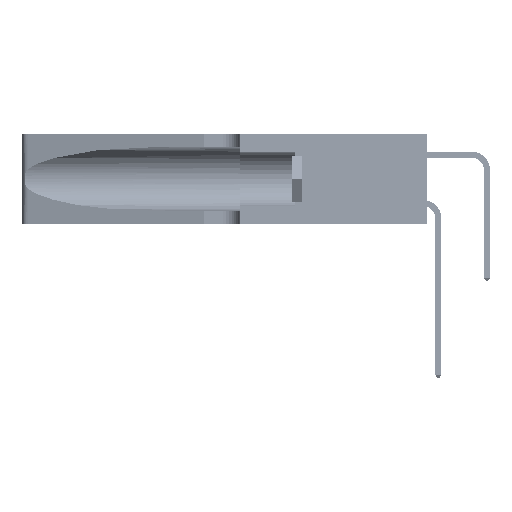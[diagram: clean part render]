
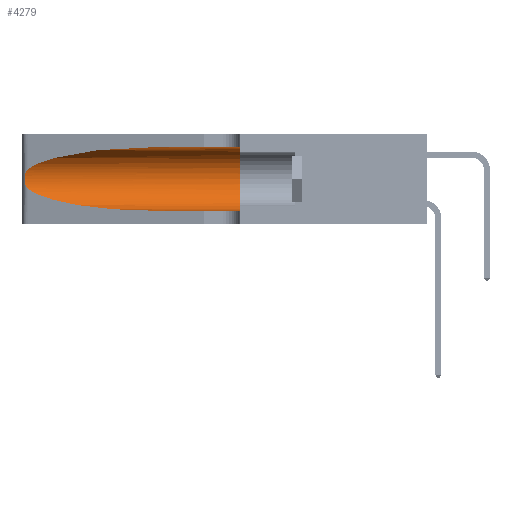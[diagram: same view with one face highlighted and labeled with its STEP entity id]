
A CAD part, left-side view. The second image highlights one B-rep face of the part: STEP entity #4279.
In plain terms, the highlighted cylindrical face has radius 3.308 mm (diameter 6.617 mm), a partial arc.
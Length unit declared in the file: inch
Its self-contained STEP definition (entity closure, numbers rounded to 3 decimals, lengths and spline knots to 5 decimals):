
#1733 = EDGE_CURVE ( 'NONE', #29096, #23608, #14990, .T. ) ;
#1966 = ORIENTED_EDGE ( 'NONE', *, *, #8866, .T. ) ;
#2706 = CARTESIAN_POINT ( 'NONE',  ( 0.25487, 1.22718, 0.22369 ) ) ;
#3504 = CARTESIAN_POINT ( 'NONE',  ( 0.25555, 1.22993, 0.14849 ) ) ;
#4279 = ADVANCED_FACE ( 'NONE', ( #16477 ), #40839, .F. ) ;
#5134 = CARTESIAN_POINT ( 'NONE',  ( 0.2373, 1.15595, 0.08982 ) ) ;
#5676 = CARTESIAN_POINT ( 'NONE',  ( 0.25487, 1.22718, 0.14631 ) ) ;
#7489 = CARTESIAN_POINT ( 'NONE',  ( 0.25487, 1.22718, 0.22369 ) ) ;
#8312 = CARTESIAN_POINT ( 'NONE',  ( 0.1305, 1.61858, 0.185 ) ) ;
#8866 = EDGE_CURVE ( 'NONE', #23500, #29096, #22328, .T. ) ;
#8928 = CARTESIAN_POINT ( 'NONE',  ( 0.1305, 0.72297, 0.05475 ) ) ;
#10269 = CARTESIAN_POINT ( 'NONE',  ( 0.25787, 1.23484, 0.2124 ) ) ;
#12177 = CARTESIAN_POINT ( 'NONE',  ( 0.1305, 0.35, 0.31525 ) ) ;
#12567 = CARTESIAN_POINT ( 'NONE',  ( 0.1305, 1.61858, 0.05475 ) ) ;
#12892 = VERTEX_POINT ( 'NONE', #12177 ) ;
#13508 = ORIENTED_EDGE ( 'NONE', *, *, #34425, .F. ) ;
#14007 = CARTESIAN_POINT ( 'NONE',  ( 0.1305, 1.61858, 0.31525 ) ) ;
#14303 = CARTESIAN_POINT ( 'NONE',  ( 0.1305, 0.35, 0.185 ) ) ;
#14594 = CARTESIAN_POINT ( 'NONE',  ( 0.26018, 1.23835, 0.19895 ) ) ;
#14990 = LINE ( 'NONE', #12567, #33189 ) ;
#16477 = FACE_OUTER_BOUND ( 'NONE', #47210, .T. ) ;
#16656 = VERTEX_POINT ( 'NONE', #23889 ) ;
#18002 = DIRECTION ( 'NONE',  ( 0., 0., 1. ) ) ;
#18304 = CARTESIAN_POINT ( 'NONE',  ( 0.26075, 1.23896, 0.178 ) ) ;
#19402 = DIRECTION ( 'NONE',  ( 0., 0., -1. ) ) ;
#21965 = CARTESIAN_POINT ( 'NONE',  ( 0.25856, 1.23593, 0.16098 ) ) ;
#22129 = CARTESIAN_POINT ( 'NONE',  ( 0.1305, 0.72297, 0.31525 ) ) ;
#22328 =( BOUNDED_CURVE ( )  B_SPLINE_CURVE ( 3, ( #30811, #5134, #23558, #8928 ),
 .UNSPECIFIED., .F., .T. ) 
 B_SPLINE_CURVE_WITH_KNOTS ( ( 4, 4 ),
 ( 3.44316, 4.71239 ),
 .UNSPECIFIED. ) 
 CURVE ( )  GEOMETRIC_REPRESENTATION_ITEM ( )  RATIONAL_B_SPLINE_CURVE ( ( 1., 0.87, 0.87, 1. ) ) 
 REPRESENTATION_ITEM ( '' )  );
#23151 = CARTESIAN_POINT ( 'NONE',  ( 0.25487, 1.22718, 0.22369 ) ) ;
#23500 = VERTEX_POINT ( 'NONE', #5676 ) ;
#23558 = CARTESIAN_POINT ( 'NONE',  ( 0.18966, 0.96281, 0.05475 ) ) ;
#23608 = VERTEX_POINT ( 'NONE', #28349 ) ;
#23634 = EDGE_CURVE ( 'NONE', #28376, #23500, #27299, .T. ) ;
#23889 = CARTESIAN_POINT ( 'NONE',  ( 0.1305, 0.72297, 0.31525 ) ) ;
#24861 = CARTESIAN_POINT ( 'NONE',  ( 0.25555, 1.22994, 0.2215 ) ) ;
#25637 = CARTESIAN_POINT ( 'NONE',  ( 0.25639, 1.23186, 0.15144 ) ) ;
#25801 = CARTESIAN_POINT ( 'NONE',  ( 0.18966, 0.96281, 0.31525 ) ) ;
#27299 = B_SPLINE_CURVE_WITH_KNOTS ( 'NONE', 3,
 ( #2706, #24861, #32103, #10269, #35726, #14594, #39980, #18304, #43600, #21965, #47193, #25637, #3504, #29287 ),
 .UNSPECIFIED., .F., .F.,
 ( 4, 2, 2, 2, 2, 2, 4 ),
 ( 0., 0.00027, 0.00053, 0.00107, 0.0016, 0.00187, 0.00214 ),
 .UNSPECIFIED. ) ;
#27392 = CARTESIAN_POINT ( 'NONE',  ( 0.1305, 0.72297, 0.05475 ) ) ;
#28349 = CARTESIAN_POINT ( 'NONE',  ( 0.1305, 0.35, 0.05475 ) ) ;
#28376 = VERTEX_POINT ( 'NONE', #23151 ) ;
#29096 = VERTEX_POINT ( 'NONE', #27392 ) ;
#29287 = CARTESIAN_POINT ( 'NONE',  ( 0.25487, 1.22718, 0.14631 ) ) ;
#29330 = VECTOR ( 'NONE', #39397, 39.37008 ) ;
#29403 = ORIENTED_EDGE ( 'NONE', *, *, #37634, .F. ) ;
#29426 = CARTESIAN_POINT ( 'NONE',  ( 0.2373, 1.15595, 0.28018 ) ) ;
#30689 = CIRCLE ( 'NONE', #37419, 0.13025 ) ;
#30811 = CARTESIAN_POINT ( 'NONE',  ( 0.25487, 1.22718, 0.14631 ) ) ;
#30992 = ORIENTED_EDGE ( 'NONE', *, *, #42796, .T. ) ;
#31978 = ORIENTED_EDGE ( 'NONE', *, *, #1733, .T. ) ;
#32103 = CARTESIAN_POINT ( 'NONE',  ( 0.25639, 1.23184, 0.21858 ) ) ;
#32977 = AXIS2_PLACEMENT_3D ( 'NONE', #8312, #41095, #19402 ) ;
#33189 = VECTOR ( 'NONE', #34338, 39.37008 ) ;
#34338 = DIRECTION ( 'NONE',  ( 0., -1., 0. ) ) ;
#34425 = EDGE_CURVE ( 'NONE', #16656, #12892, #38916, .T. ) ;
#35726 = CARTESIAN_POINT ( 'NONE',  ( 0.25854, 1.2359, 0.20912 ) ) ;
#37419 = AXIS2_PLACEMENT_3D ( 'NONE', #14303, #39686, #18002 ) ;
#37634 = EDGE_CURVE ( 'NONE', #12892, #23608, #30689, .T. ) ;
#38916 = LINE ( 'NONE', #14007, #29330 ) ;
#39397 = DIRECTION ( 'NONE',  ( 0., -1., 0. ) ) ;
#39686 = DIRECTION ( 'NONE',  ( 0., 1., 0. ) ) ;
#39980 = CARTESIAN_POINT ( 'NONE',  ( 0.26075, 1.23896, 0.19203 ) ) ;
#40839 = CYLINDRICAL_SURFACE ( 'NONE', #32977, 0.13025 ) ;
#41095 = DIRECTION ( 'NONE',  ( 0., -1., 0. ) ) ;
#42796 = EDGE_CURVE ( 'NONE', #16656, #28376, #45455, .T. ) ;
#43600 = CARTESIAN_POINT ( 'NONE',  ( 0.26017, 1.23833, 0.17102 ) ) ;
#44501 = ORIENTED_EDGE ( 'NONE', *, *, #23634, .T. ) ;
#45455 =( BOUNDED_CURVE ( )  B_SPLINE_CURVE ( 3, ( #22129, #25801, #29426, #7489 ),
 .UNSPECIFIED., .F., .F. ) 
 B_SPLINE_CURVE_WITH_KNOTS ( ( 4, 4 ),
 ( 1.5708, 2.84003 ),
 .UNSPECIFIED. ) 
 CURVE ( )  GEOMETRIC_REPRESENTATION_ITEM ( )  RATIONAL_B_SPLINE_CURVE ( ( 1., 0.87, 0.87, 1. ) ) 
 REPRESENTATION_ITEM ( '' )  );
#47193 = CARTESIAN_POINT ( 'NONE',  ( 0.25789, 1.23486, 0.15765 ) ) ;
#47210 = EDGE_LOOP ( 'NONE', ( #30992, #44501, #1966, #31978, #29403, #13508 ) ) ;
